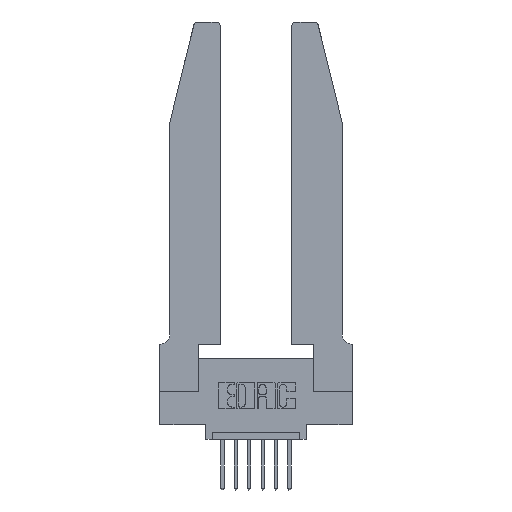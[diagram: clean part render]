
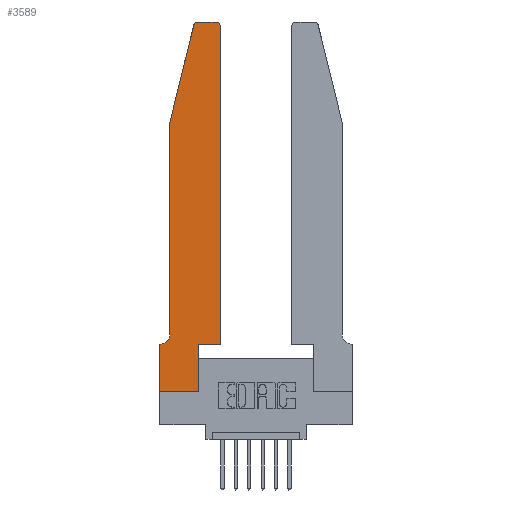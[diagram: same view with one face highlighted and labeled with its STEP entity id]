
A CAD part, top view. The second image highlights one B-rep face of the part: STEP entity #3589.
In plain terms, the highlighted planar face has unit normal (0, 0, 1).
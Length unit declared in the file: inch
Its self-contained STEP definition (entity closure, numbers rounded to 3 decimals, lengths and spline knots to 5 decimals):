
#17 = CARTESIAN_POINT ( 'NONE',  ( 0.2865, 0., 0.37 ) ) ;
#19 = ORIENTED_EDGE ( 'NONE', *, *, #7426, .T. ) ;
#348 = VERTEX_POINT ( 'NONE', #3837 ) ;
#468 = VECTOR ( 'NONE', #11581, 39.37008 ) ;
#591 = EDGE_CURVE ( 'NONE', #8579, #4783, #6540, .T. ) ;
#602 = EDGE_CURVE ( 'NONE', #5465, #1682, #11535, .T. ) ;
#649 = CARTESIAN_POINT ( 'NONE',  ( 0., 0., 0.37 ) ) ;
#752 = FACE_OUTER_BOUND ( 'NONE', #3149, .T. ) ;
#801 = VECTOR ( 'NONE', #8632, 39.37008 ) ;
#1236 = EDGE_CURVE ( 'NONE', #4783, #1830, #5136, .T. ) ;
#1273 = DIRECTION ( 'NONE',  ( 0., 0., -1. ) ) ;
#1500 = ORIENTED_EDGE ( 'NONE', *, *, #591, .T. ) ;
#1651 = CARTESIAN_POINT ( 'NONE',  ( 0.25487, 2.72718, 0.37 ) ) ;
#1682 = VERTEX_POINT ( 'NONE', #11860 ) ;
#1701 = EDGE_CURVE ( 'NONE', #3506, #7458, #6160, .T. ) ;
#1830 = VERTEX_POINT ( 'NONE', #2728 ) ;
#1927 = EDGE_CURVE ( 'NONE', #1830, #10997, #12357, .T. ) ;
#1997 = AXIS2_PLACEMENT_3D ( 'NONE', #11365, #5922, #10201 ) ;
#2002 = DIRECTION ( 'NONE',  ( 1., 0., 0. ) ) ;
#2178 = VERTEX_POINT ( 'NONE', #12036 ) ;
#2382 = DIRECTION ( 'NONE',  ( -1., 0., 0. ) ) ;
#2728 = CARTESIAN_POINT ( 'NONE',  ( 0.4505, 2.72, 0.37 ) ) ;
#2748 = VERTEX_POINT ( 'NONE', #13374 ) ;
#2830 = EDGE_CURVE ( 'NONE', #10997, #348, #4408, .T. ) ;
#3097 = LINE ( 'NONE', #5504, #6894 ) ;
#3100 = DIRECTION ( 'NONE',  ( 0., 1., 0. ) ) ;
#3149 = EDGE_LOOP ( 'NONE', ( #9564, #9108, #6045, #19, #6876, #5482, #9873, #9117, #8493, #1500, #7045, #4862 ) ) ;
#3380 = LINE ( 'NONE', #11701, #801 ) ;
#3389 = LINE ( 'NONE', #8237, #468 ) ;
#3506 = VERTEX_POINT ( 'NONE', #1651 ) ;
#3589 = ADVANCED_FACE ( 'NONE', ( #752 ), #4548, .T. ) ;
#3693 = CARTESIAN_POINT ( 'NONE',  ( 0.0055, 0.42, 0.37 ) ) ;
#3837 = CARTESIAN_POINT ( 'NONE',  ( 0.284, 2.75, 0.37 ) ) ;
#3914 = EDGE_CURVE ( 'NONE', #2748, #2178, #7114, .T. ) ;
#4408 = LINE ( 'NONE', #4958, #6981 ) ;
#4548 = PLANE ( 'NONE',  #1997 ) ;
#4555 = DIRECTION ( 'NONE',  ( 0., 1., 0. ) ) ;
#4783 = VERTEX_POINT ( 'NONE', #6688 ) ;
#4862 = ORIENTED_EDGE ( 'NONE', *, *, #1927, .T. ) ;
#4958 = CARTESIAN_POINT ( 'NONE',  ( 0.2605, 2.75, 0.37 ) ) ;
#5110 = AXIS2_PLACEMENT_3D ( 'NONE', #3693, #1273, #2382 ) ;
#5136 = LINE ( 'NONE', #10750, #8394 ) ;
#5264 = DIRECTION ( 'NONE',  ( -0.239, -0.971, 0. ) ) ;
#5301 = CARTESIAN_POINT ( 'NONE',  ( 0.0755, 0.42, 0.37 ) ) ;
#5339 = CARTESIAN_POINT ( 'NONE',  ( 0.284, 2.72, 0.37 ) ) ;
#5396 = DIRECTION ( 'NONE',  ( 0., 0., 1. ) ) ;
#5465 = VERTEX_POINT ( 'NONE', #5301 ) ;
#5482 = ORIENTED_EDGE ( 'NONE', *, *, #14251, .T. ) ;
#5504 = CARTESIAN_POINT ( 'NONE',  ( 0., 0., 0.37 ) ) ;
#5922 = DIRECTION ( 'NONE',  ( 0., 0., 1. ) ) ;
#6045 = ORIENTED_EDGE ( 'NONE', *, *, #1701, .T. ) ;
#6160 = LINE ( 'NONE', #14039, #7009 ) ;
#6540 = LINE ( 'NONE', #13398, #8580 ) ;
#6688 = CARTESIAN_POINT ( 'NONE',  ( 0.4505, 0.35, 0.37 ) ) ;
#6876 = ORIENTED_EDGE ( 'NONE', *, *, #602, .T. ) ;
#6894 = VECTOR ( 'NONE', #7706, 39.37008 ) ;
#6981 = VECTOR ( 'NONE', #8085, 39.37008 ) ;
#7009 = VECTOR ( 'NONE', #5264, 39.37008 ) ;
#7045 = ORIENTED_EDGE ( 'NONE', *, *, #1236, .T. ) ;
#7112 = EDGE_CURVE ( 'NONE', #348, #3506, #9228, .T. ) ;
#7114 = LINE ( 'NONE', #649, #11776 ) ;
#7426 = EDGE_CURVE ( 'NONE', #7458, #5465, #3380, .T. ) ;
#7458 = VERTEX_POINT ( 'NONE', #10856 ) ;
#7706 = DIRECTION ( 'NONE',  ( 1., 0., 0. ) ) ;
#8085 = DIRECTION ( 'NONE',  ( -1., 0., 0. ) ) ;
#8237 = CARTESIAN_POINT ( 'NONE',  ( 0.0755, 0.35, 0.37 ) ) ;
#8285 = VERTEX_POINT ( 'NONE', #17 ) ;
#8394 = VECTOR ( 'NONE', #3100, 39.37008 ) ;
#8493 = ORIENTED_EDGE ( 'NONE', *, *, #11276, .T. ) ;
#8517 = DIRECTION ( 'NONE',  ( 1., 0., 0. ) ) ;
#8579 = VERTEX_POINT ( 'NONE', #9436 ) ;
#8580 = VECTOR ( 'NONE', #12416, 39.37008 ) ;
#8632 = DIRECTION ( 'NONE',  ( 0., -1., 0. ) ) ;
#8941 = CARTESIAN_POINT ( 'NONE',  ( 0.2865, 0.35, 0.37 ) ) ;
#9108 = ORIENTED_EDGE ( 'NONE', *, *, #7112, .T. ) ;
#9117 = ORIENTED_EDGE ( 'NONE', *, *, #11736, .T. ) ;
#9228 = CIRCLE ( 'NONE', #11552, 0.03 ) ;
#9391 = DIRECTION ( 'NONE',  ( 0., -1., 0. ) ) ;
#9436 = CARTESIAN_POINT ( 'NONE',  ( 0.2865, 0.35, 0.37 ) ) ;
#9564 = ORIENTED_EDGE ( 'NONE', *, *, #2830, .T. ) ;
#9873 = ORIENTED_EDGE ( 'NONE', *, *, #3914, .T. ) ;
#10201 = DIRECTION ( 'NONE',  ( 1., 0., 0. ) ) ;
#10325 = LINE ( 'NONE', #8941, #14113 ) ;
#10750 = CARTESIAN_POINT ( 'NONE',  ( 0.4505, 0.35, 0.37 ) ) ;
#10856 = CARTESIAN_POINT ( 'NONE',  ( 0.0755, 2., 0.37 ) ) ;
#10997 = VERTEX_POINT ( 'NONE', #12787 ) ;
#11212 = AXIS2_PLACEMENT_3D ( 'NONE', #11902, #13048, #8517 ) ;
#11276 = EDGE_CURVE ( 'NONE', #8285, #8579, #10325, .T. ) ;
#11365 = CARTESIAN_POINT ( 'NONE',  ( 0., 0.35, 0.37 ) ) ;
#11535 = CIRCLE ( 'NONE', #5110, 0.07 ) ;
#11552 = AXIS2_PLACEMENT_3D ( 'NONE', #5339, #5396, #2002 ) ;
#11581 = DIRECTION ( 'NONE',  ( -1., 0., 0. ) ) ;
#11701 = CARTESIAN_POINT ( 'NONE',  ( 0.0755, 2., 0.37 ) ) ;
#11736 = EDGE_CURVE ( 'NONE', #2178, #8285, #3097, .T. ) ;
#11776 = VECTOR ( 'NONE', #9391, 39.37008 ) ;
#11860 = CARTESIAN_POINT ( 'NONE',  ( 0.0055, 0.35, 0.37 ) ) ;
#11902 = CARTESIAN_POINT ( 'NONE',  ( 0.4205, 2.72, 0.37 ) ) ;
#12036 = CARTESIAN_POINT ( 'NONE',  ( 0., 0., 0.37 ) ) ;
#12357 = CIRCLE ( 'NONE', #11212, 0.03 ) ;
#12416 = DIRECTION ( 'NONE',  ( 1., 0., 0. ) ) ;
#12787 = CARTESIAN_POINT ( 'NONE',  ( 0.4205, 2.75, 0.37 ) ) ;
#13048 = DIRECTION ( 'NONE',  ( 0., 0., 1. ) ) ;
#13374 = CARTESIAN_POINT ( 'NONE',  ( 0., 0.35, 0.37 ) ) ;
#13398 = CARTESIAN_POINT ( 'NONE',  ( 0.4505, 0.35, 0.37 ) ) ;
#14039 = CARTESIAN_POINT ( 'NONE',  ( 0.0755, 2., 0.37 ) ) ;
#14113 = VECTOR ( 'NONE', #4555, 39.37008 ) ;
#14251 = EDGE_CURVE ( 'NONE', #1682, #2748, #3389, .T. ) ;
